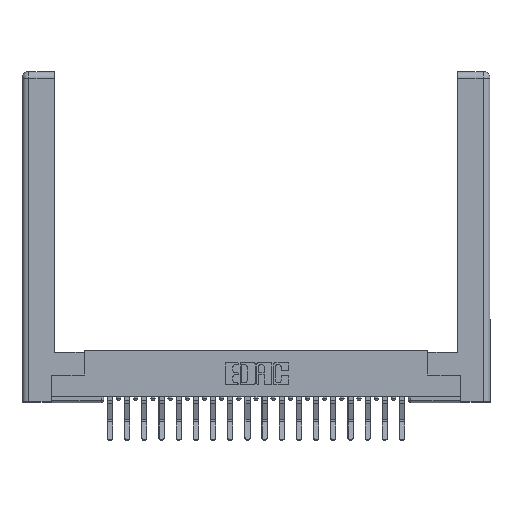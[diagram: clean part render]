
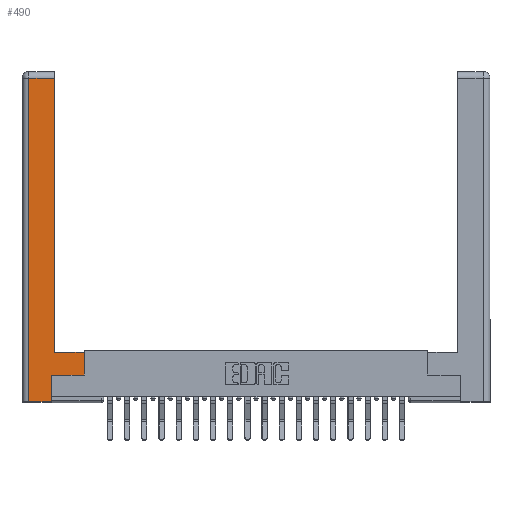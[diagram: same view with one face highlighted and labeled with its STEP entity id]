
A CAD part, top view. The second image highlights one B-rep face of the part: STEP entity #490.
In plain terms, the highlighted planar face has unit normal (0, 0, 1).
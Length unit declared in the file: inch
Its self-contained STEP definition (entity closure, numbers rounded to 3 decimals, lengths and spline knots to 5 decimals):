
#83 = DIRECTION ( 'NONE',  ( 1., 0., 0. ) ) ;
#490 = ADVANCED_FACE ( 'NONE', ( #16925 ), #14670, .F. ) ;
#831 = LINE ( 'NONE', #18120, #13114 ) ;
#1034 = EDGE_CURVE ( 'NONE', #7284, #2032, #6361, .T. ) ;
#1280 = VERTEX_POINT ( 'NONE', #15178 ) ;
#1817 = VERTEX_POINT ( 'NONE', #15379 ) ;
#2032 = VERTEX_POINT ( 'NONE', #7874 ) ;
#2986 = DIRECTION ( 'NONE',  ( 1., 0., 0. ) ) ;
#3108 = CARTESIAN_POINT ( 'NONE',  ( 0.565, 0.245, 0. ) ) ;
#4466 = EDGE_CURVE ( 'NONE', #6304, #1280, #831, .T. ) ;
#4673 = DIRECTION ( 'NONE',  ( 0., 0., -1. ) ) ;
#4942 = EDGE_LOOP ( 'NONE', ( #9452, #13614, #19829, #11321, #21453, #10107, #16763, #5996 ) ) ;
#5085 = DIRECTION ( 'NONE',  ( 0., 1., 0. ) ) ;
#5496 = CARTESIAN_POINT ( 'NONE',  ( 0.0615, 2.94, 0. ) ) ;
#5643 = CARTESIAN_POINT ( 'NONE',  ( 0.565, 0.45, 0. ) ) ;
#5793 = LINE ( 'NONE', #7876, #7619 ) ;
#5996 = ORIENTED_EDGE ( 'NONE', *, *, #11018, .T. ) ;
#6304 = VERTEX_POINT ( 'NONE', #11624 ) ;
#6361 = LINE ( 'NONE', #12980, #12944 ) ;
#7284 = VERTEX_POINT ( 'NONE', #16010 ) ;
#7384 = CARTESIAN_POINT ( 'NONE',  ( 0.565, 0.245, 0. ) ) ;
#7473 = VECTOR ( 'NONE', #17396, 39.37008 ) ;
#7619 = VECTOR ( 'NONE', #12741, 39.37008 ) ;
#7874 = CARTESIAN_POINT ( 'NONE',  ( 0.265, 0.245, 0. ) ) ;
#7876 = CARTESIAN_POINT ( 'NONE',  ( 0.295, 0.45, 0. ) ) ;
#8045 = DIRECTION ( 'NONE',  ( 0., -1., 0. ) ) ;
#8304 = CARTESIAN_POINT ( 'NONE',  ( 0.295, 3., 0. ) ) ;
#8734 = VECTOR ( 'NONE', #2986, 39.37008 ) ;
#9369 = VECTOR ( 'NONE', #83, 39.37008 ) ;
#9452 = ORIENTED_EDGE ( 'NONE', *, *, #10891, .T. ) ;
#9917 = CARTESIAN_POINT ( 'NONE',  ( 0.265, 0., 0. ) ) ;
#10107 = ORIENTED_EDGE ( 'NONE', *, *, #17612, .T. ) ;
#10251 = LINE ( 'NONE', #8304, #17892 ) ;
#10891 = EDGE_CURVE ( 'NONE', #13189, #1817, #10251, .T. ) ;
#11018 = EDGE_CURVE ( 'NONE', #15495, #13189, #5793, .T. ) ;
#11321 = ORIENTED_EDGE ( 'NONE', *, *, #13102, .T. ) ;
#11488 = LINE ( 'NONE', #5496, #15426 ) ;
#11624 = CARTESIAN_POINT ( 'NONE',  ( 0.0615, 2.94, 0. ) ) ;
#12193 = LINE ( 'NONE', #5643, #7473 ) ;
#12308 = DIRECTION ( 'NONE',  ( -1., 0., 0. ) ) ;
#12741 = DIRECTION ( 'NONE',  ( -1., 0., 0. ) ) ;
#12944 = VECTOR ( 'NONE', #13060, 39.37008 ) ;
#12980 = CARTESIAN_POINT ( 'NONE',  ( 0.265, 0.245, 0. ) ) ;
#13060 = DIRECTION ( 'NONE',  ( 0., 1., 0. ) ) ;
#13082 = CARTESIAN_POINT ( 'NONE',  ( 0., 0., 0. ) ) ;
#13102 = EDGE_CURVE ( 'NONE', #1280, #7284, #13830, .T. ) ;
#13114 = VECTOR ( 'NONE', #8045, 39.37008 ) ;
#13189 = VERTEX_POINT ( 'NONE', #20078 ) ;
#13236 = LINE ( 'NONE', #7384, #8734 ) ;
#13614 = ORIENTED_EDGE ( 'NONE', *, *, #15294, .T. ) ;
#13830 = LINE ( 'NONE', #9917, #9369 ) ;
#14670 = PLANE ( 'NONE',  #15139 ) ;
#15139 = AXIS2_PLACEMENT_3D ( 'NONE', #13082, #4673, #18391 ) ;
#15178 = CARTESIAN_POINT ( 'NONE',  ( 0.0615, 0., 0. ) ) ;
#15294 = EDGE_CURVE ( 'NONE', #1817, #6304, #11488, .T. ) ;
#15379 = CARTESIAN_POINT ( 'NONE',  ( 0.295, 2.94, 0. ) ) ;
#15426 = VECTOR ( 'NONE', #12308, 39.37008 ) ;
#15495 = VERTEX_POINT ( 'NONE', #18196 ) ;
#16010 = CARTESIAN_POINT ( 'NONE',  ( 0.265, 0., 0. ) ) ;
#16475 = VERTEX_POINT ( 'NONE', #3108 ) ;
#16763 = ORIENTED_EDGE ( 'NONE', *, *, #17514, .T. ) ;
#16925 = FACE_OUTER_BOUND ( 'NONE', #4942, .T. ) ;
#17396 = DIRECTION ( 'NONE',  ( 0., 1., 0. ) ) ;
#17514 = EDGE_CURVE ( 'NONE', #16475, #15495, #12193, .T. ) ;
#17612 = EDGE_CURVE ( 'NONE', #2032, #16475, #13236, .T. ) ;
#17892 = VECTOR ( 'NONE', #5085, 39.37008 ) ;
#18120 = CARTESIAN_POINT ( 'NONE',  ( 0.0615, 0., 0. ) ) ;
#18196 = CARTESIAN_POINT ( 'NONE',  ( 0.565, 0.45, 0. ) ) ;
#18391 = DIRECTION ( 'NONE',  ( -1., 0., 0. ) ) ;
#19829 = ORIENTED_EDGE ( 'NONE', *, *, #4466, .T. ) ;
#20078 = CARTESIAN_POINT ( 'NONE',  ( 0.295, 0.45, 0. ) ) ;
#21453 = ORIENTED_EDGE ( 'NONE', *, *, #1034, .T. ) ;
